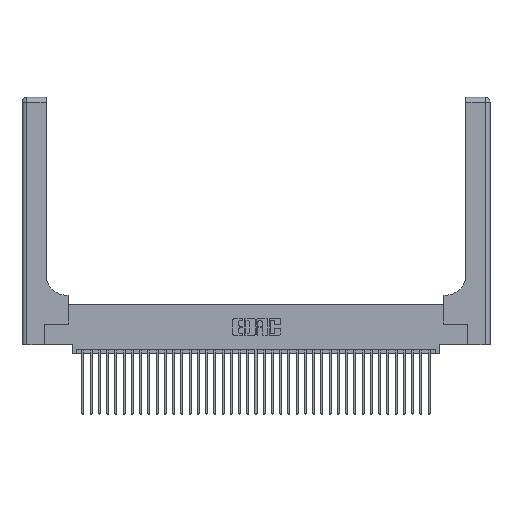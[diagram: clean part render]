
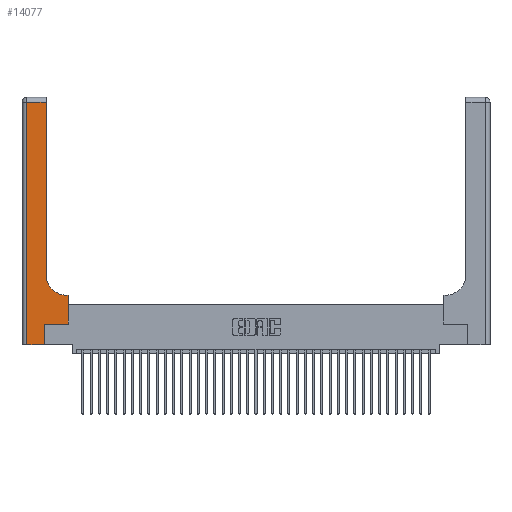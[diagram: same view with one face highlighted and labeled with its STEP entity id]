
A CAD part, top view. The second image highlights one B-rep face of the part: STEP entity #14077.
In plain terms, the highlighted planar face has unit normal (0, 0, 1).
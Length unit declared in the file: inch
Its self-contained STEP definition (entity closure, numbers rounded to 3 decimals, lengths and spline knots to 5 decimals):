
#897 = ORIENTED_EDGE ( 'NONE', *, *, #28707, .T. ) ;
#1282 = DIRECTION ( 'NONE',  ( 1., 0., 0. ) ) ;
#2006 = EDGE_CURVE ( 'NONE', #27246, #22993, #24509, .T. ) ;
#2077 = EDGE_CURVE ( 'NONE', #9865, #26131, #37603, .T. ) ;
#2166 = AXIS2_PLACEMENT_3D ( 'NONE', #3266, #24389, #6318 ) ;
#3014 = EDGE_CURVE ( 'NONE', #14488, #26782, #14075, .T. ) ;
#3266 = CARTESIAN_POINT ( 'NONE',  ( 0.5415, 0.85, 0.37 ) ) ;
#3499 = PLANE ( 'NONE',  #32480 ) ;
#3728 = CARTESIAN_POINT ( 'NONE',  ( 0.2915, 3., 0.37 ) ) ;
#3753 = ORIENTED_EDGE ( 'NONE', *, *, #2006, .T. ) ;
#3799 = VECTOR ( 'NONE', #7672, 39.37008 ) ;
#3807 = CARTESIAN_POINT ( 'NONE',  ( 0.269, 0.25, 0.37 ) ) ;
#4623 = CARTESIAN_POINT ( 'NONE',  ( 0.06, 2.94, 0.37 ) ) ;
#5173 = ORIENTED_EDGE ( 'NONE', *, *, #5804, .T. ) ;
#5804 = EDGE_CURVE ( 'NONE', #24497, #14488, #17283, .T. ) ;
#6083 = VECTOR ( 'NONE', #15926, 39.37008 ) ;
#6294 = CARTESIAN_POINT ( 'NONE',  ( 0.5415, 0.6, 0.37 ) ) ;
#6318 = DIRECTION ( 'NONE',  ( 1., 0., 0. ) ) ;
#7048 = ORIENTED_EDGE ( 'NONE', *, *, #3014, .T. ) ;
#7672 = DIRECTION ( 'NONE',  ( 0., -1., 0. ) ) ;
#7882 = CARTESIAN_POINT ( 'NONE',  ( 0.2915, 0.85, 0.37 ) ) ;
#8192 = FACE_OUTER_BOUND ( 'NONE', #38071, .T. ) ;
#9594 = CARTESIAN_POINT ( 'NONE',  ( 0., 2.94, 0.37 ) ) ;
#9865 = VERTEX_POINT ( 'NONE', #19503 ) ;
#12583 = LINE ( 'NONE', #28460, #35632 ) ;
#12728 = CARTESIAN_POINT ( 'NONE',  ( 0., 3., 0.37 ) ) ;
#13611 = VECTOR ( 'NONE', #33793, 39.37008 ) ;
#14075 = LINE ( 'NONE', #24903, #6083 ) ;
#14077 = ADVANCED_FACE ( 'NONE', ( #8192 ), #3499, .F. ) ;
#14403 = DIRECTION ( 'NONE',  ( 1., 0., 0. ) ) ;
#14488 = VERTEX_POINT ( 'NONE', #38568 ) ;
#15468 = VECTOR ( 'NONE', #33859, 39.37008 ) ;
#15772 = DIRECTION ( 'NONE',  ( 0., 0., -1. ) ) ;
#15926 = DIRECTION ( 'NONE',  ( 0., 1., 0. ) ) ;
#16492 = LINE ( 'NONE', #22428, #31542 ) ;
#17283 = LINE ( 'NONE', #38436, #28125 ) ;
#17456 = ORIENTED_EDGE ( 'NONE', *, *, #29634, .T. ) ;
#17485 = EDGE_CURVE ( 'NONE', #21307, #27246, #12583, .T. ) ;
#17961 = VERTEX_POINT ( 'NONE', #32747 ) ;
#18587 = EDGE_CURVE ( 'NONE', #17961, #21307, #37453, .T. ) ;
#19503 = CARTESIAN_POINT ( 'NONE',  ( 0.2915, 2.94, 0.37 ) ) ;
#21307 = VERTEX_POINT ( 'NONE', #32893 ) ;
#21545 = VECTOR ( 'NONE', #29560, 39.37008 ) ;
#22428 = CARTESIAN_POINT ( 'NONE',  ( 0.269, 0.25, 0.37 ) ) ;
#22993 = VERTEX_POINT ( 'NONE', #7882 ) ;
#24389 = DIRECTION ( 'NONE',  ( 0., 0., -1. ) ) ;
#24497 = VERTEX_POINT ( 'NONE', #34054 ) ;
#24509 = CIRCLE ( 'NONE', #2166, 0.25 ) ;
#24903 = CARTESIAN_POINT ( 'NONE',  ( 0.269, 0., 0.37 ) ) ;
#24998 = ORIENTED_EDGE ( 'NONE', *, *, #18587, .T. ) ;
#26131 = VERTEX_POINT ( 'NONE', #4623 ) ;
#26402 = ORIENTED_EDGE ( 'NONE', *, *, #2077, .T. ) ;
#26552 = CARTESIAN_POINT ( 'NONE',  ( 0.5585, 0.25, 0.37 ) ) ;
#26782 = VERTEX_POINT ( 'NONE', #3807 ) ;
#27246 = VERTEX_POINT ( 'NONE', #6294 ) ;
#28125 = VECTOR ( 'NONE', #14403, 39.37008 ) ;
#28287 = ORIENTED_EDGE ( 'NONE', *, *, #31677, .T. ) ;
#28460 = CARTESIAN_POINT ( 'NONE',  ( 0.2915, 0.6, 0.37 ) ) ;
#28707 = EDGE_CURVE ( 'NONE', #26782, #17961, #16492, .T. ) ;
#28777 = CARTESIAN_POINT ( 'NONE',  ( 0.06, 3., 0.37 ) ) ;
#29560 = DIRECTION ( 'NONE',  ( 0., 1., 0. ) ) ;
#29634 = EDGE_CURVE ( 'NONE', #22993, #9865, #31473, .T. ) ;
#31471 = DIRECTION ( 'NONE',  ( -1., 0., 0. ) ) ;
#31473 = LINE ( 'NONE', #3728, #15468 ) ;
#31542 = VECTOR ( 'NONE', #1282, 39.37008 ) ;
#31677 = EDGE_CURVE ( 'NONE', #26131, #24497, #35833, .T. ) ;
#32480 = AXIS2_PLACEMENT_3D ( 'NONE', #12728, #15772, #36778 ) ;
#32747 = CARTESIAN_POINT ( 'NONE',  ( 0.5585, 0.25, 0.37 ) ) ;
#32893 = CARTESIAN_POINT ( 'NONE',  ( 0.5585, 0.6, 0.37 ) ) ;
#33793 = DIRECTION ( 'NONE',  ( -1., 0., 0. ) ) ;
#33859 = DIRECTION ( 'NONE',  ( 0., 1., 0. ) ) ;
#33883 = ORIENTED_EDGE ( 'NONE', *, *, #17485, .T. ) ;
#34054 = CARTESIAN_POINT ( 'NONE',  ( 0.06, 0., 0.37 ) ) ;
#35632 = VECTOR ( 'NONE', #31471, 39.37008 ) ;
#35833 = LINE ( 'NONE', #28777, #3799 ) ;
#36778 = DIRECTION ( 'NONE',  ( -1., 0., 0. ) ) ;
#37453 = LINE ( 'NONE', #26552, #21545 ) ;
#37603 = LINE ( 'NONE', #9594, #13611 ) ;
#38071 = EDGE_LOOP ( 'NONE', ( #17456, #26402, #28287, #5173, #7048, #897, #24998, #33883, #3753 ) ) ;
#38436 = CARTESIAN_POINT ( 'NONE',  ( 0., 0., 0.37 ) ) ;
#38568 = CARTESIAN_POINT ( 'NONE',  ( 0.269, 0., 0.37 ) ) ;
